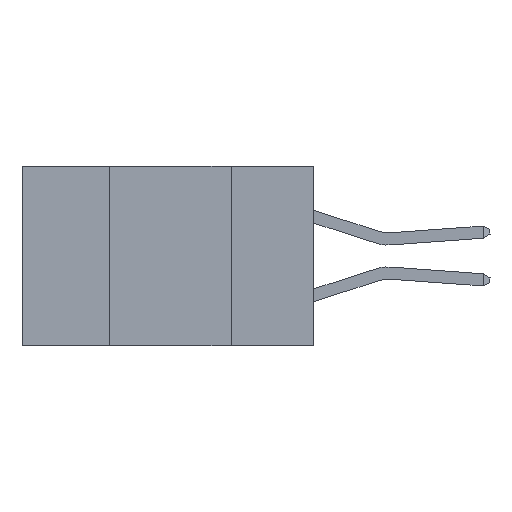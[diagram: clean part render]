
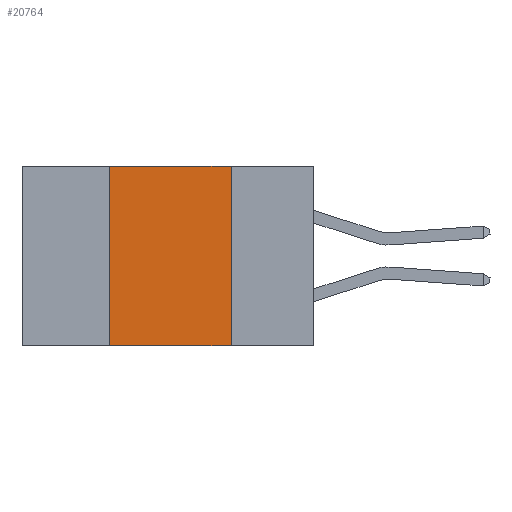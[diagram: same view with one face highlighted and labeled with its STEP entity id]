
A CAD part, left-side view. The second image highlights one B-rep face of the part: STEP entity #20764.
In plain terms, the highlighted planar face has unit normal (-1, 0, 0).
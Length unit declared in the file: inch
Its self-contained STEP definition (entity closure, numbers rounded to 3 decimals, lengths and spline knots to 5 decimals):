
#205 = CARTESIAN_POINT ( 'NONE',  ( 0., 0.17, 0. ) ) ;
#568 = ORIENTED_EDGE ( 'NONE', *, *, #6893, .F. ) ;
#642 = ORIENTED_EDGE ( 'NONE', *, *, #20114, .F. ) ;
#1032 = CARTESIAN_POINT ( 'NONE',  ( 0., 0.6, 0. ) ) ;
#1253 = VERTEX_POINT ( 'NONE', #9894 ) ;
#1606 = EDGE_CURVE ( 'NONE', #2945, #1253, #7701, .T. ) ;
#2945 = VERTEX_POINT ( 'NONE', #205 ) ;
#3203 = CARTESIAN_POINT ( 'NONE',  ( 0., 0.42, -0.37 ) ) ;
#3773 = LINE ( 'NONE', #18734, #11844 ) ;
#4331 = DIRECTION ( 'NONE',  ( 1., 0., 0. ) ) ;
#6143 = EDGE_LOOP ( 'NONE', ( #6326, #642, #568, #6948 ) ) ;
#6326 = ORIENTED_EDGE ( 'NONE', *, *, #1606, .F. ) ;
#6893 = EDGE_CURVE ( 'NONE', #7742, #20552, #12683, .T. ) ;
#6948 = ORIENTED_EDGE ( 'NONE', *, *, #18206, .T. ) ;
#7484 = PLANE ( 'NONE',  #15992 ) ;
#7701 = LINE ( 'NONE', #16753, #15761 ) ;
#7742 = VERTEX_POINT ( 'NONE', #3203 ) ;
#9123 = DIRECTION ( 'NONE',  ( 0., -1., 0. ) ) ;
#9153 = CARTESIAN_POINT ( 'NONE',  ( 0., 0.42, 0. ) ) ;
#9890 = VECTOR ( 'NONE', #13961, 39.37008 ) ;
#9894 = CARTESIAN_POINT ( 'NONE',  ( 0., 0.17, -0.37 ) ) ;
#10216 = CARTESIAN_POINT ( 'NONE',  ( 0., 0.42, 0. ) ) ;
#11844 = VECTOR ( 'NONE', #9123, 39.37008 ) ;
#12602 = DIRECTION ( 'NONE',  ( 0., 0., -1. ) ) ;
#12683 = LINE ( 'NONE', #9153, #9890 ) ;
#13961 = DIRECTION ( 'NONE',  ( 0., 0., 1. ) ) ;
#14932 = VECTOR ( 'NONE', #20330, 39.37008 ) ;
#15425 = LINE ( 'NONE', #18730, #14932 ) ;
#15571 = DIRECTION ( 'NONE',  ( 0., 0., -1. ) ) ;
#15761 = VECTOR ( 'NONE', #12602, 39.37008 ) ;
#15992 = AXIS2_PLACEMENT_3D ( 'NONE', #1032, #4331, #15571 ) ;
#16753 = CARTESIAN_POINT ( 'NONE',  ( 0., 0.17, 0. ) ) ;
#18206 = EDGE_CURVE ( 'NONE', #7742, #1253, #15425, .T. ) ;
#18730 = CARTESIAN_POINT ( 'NONE',  ( 0., 0.6, -0.37 ) ) ;
#18734 = CARTESIAN_POINT ( 'NONE',  ( 0., 0.6, 0. ) ) ;
#20038 = FACE_OUTER_BOUND ( 'NONE', #6143, .T. ) ;
#20114 = EDGE_CURVE ( 'NONE', #20552, #2945, #3773, .T. ) ;
#20330 = DIRECTION ( 'NONE',  ( 0., -1., 0. ) ) ;
#20552 = VERTEX_POINT ( 'NONE', #10216 ) ;
#20764 = ADVANCED_FACE ( 'NONE', ( #20038 ), #7484, .F. ) ;
